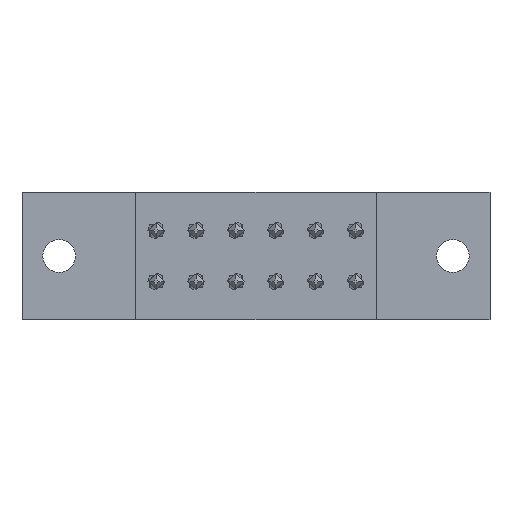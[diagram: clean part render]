
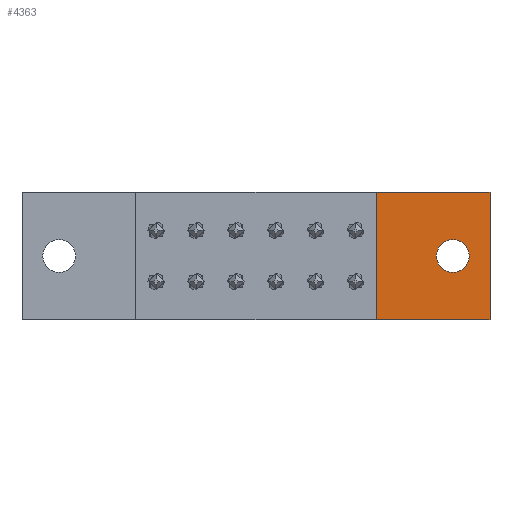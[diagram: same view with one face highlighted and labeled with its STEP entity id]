
A CAD part, front view. The second image highlights one B-rep face of the part: STEP entity #4363.
In plain terms, the highlighted planar face has unit normal (0, -1, 0).
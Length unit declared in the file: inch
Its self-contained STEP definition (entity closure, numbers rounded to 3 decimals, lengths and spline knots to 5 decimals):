
#389 = VERTEX_POINT ( 'NONE', #486 ) ;
#486 = CARTESIAN_POINT ( 'NONE',  ( 1.385, 0.163, 0. ) ) ;
#1177 = VECTOR ( 'NONE', #9337, 39.37008 ) ;
#1656 = ORIENTED_EDGE ( 'NONE', *, *, #9007, .T. ) ;
#1681 = LINE ( 'NONE', #3492, #4332 ) ;
#1894 = DIRECTION ( 'NONE',  ( 0., 0., -1. ) ) ;
#2116 = VERTEX_POINT ( 'NONE', #6419 ) ;
#2620 = VECTOR ( 'NONE', #1894, 39.37008 ) ;
#2778 = AXIS2_PLACEMENT_3D ( 'NONE', #4044, #10403, #4236 ) ;
#3349 = LINE ( 'NONE', #5354, #1177 ) ;
#3492 = CARTESIAN_POINT ( 'NONE',  ( 1.83, 0.163, -0.5 ) ) ;
#3791 = CARTESIAN_POINT ( 'NONE',  ( 1.6845, 0.163, -0.186 ) ) ;
#4044 = CARTESIAN_POINT ( 'NONE',  ( 1.6845, 0.163, -0.25 ) ) ;
#4084 = LINE ( 'NONE', #6228, #2620 ) ;
#4207 = VERTEX_POINT ( 'NONE', #5032 ) ;
#4236 = DIRECTION ( 'NONE',  ( 0., 0., -1. ) ) ;
#4332 = VECTOR ( 'NONE', #6622, 39.37008 ) ;
#4359 = CARTESIAN_POINT ( 'NONE',  ( 1.83, 0.163, 0. ) ) ;
#4363 = ADVANCED_FACE ( 'NONE', ( #11384, #7287 ), #12642, .T. ) ;
#5032 = CARTESIAN_POINT ( 'NONE',  ( 1.6845, 0.163, -0.314 ) ) ;
#5340 = DIRECTION ( 'NONE',  ( 1., 0., 0. ) ) ;
#5354 = CARTESIAN_POINT ( 'NONE',  ( 1.83, 0.163, 0. ) ) ;
#5498 = EDGE_CURVE ( 'NONE', #2116, #389, #3349, .T. ) ;
#6051 = EDGE_CURVE ( 'NONE', #7938, #4207, #7603, .T. ) ;
#6228 = CARTESIAN_POINT ( 'NONE',  ( 1.385, 0.163, -0.5 ) ) ;
#6338 = ORIENTED_EDGE ( 'NONE', *, *, #12114, .T. ) ;
#6344 = DIRECTION ( 'NONE',  ( 0., -1., 0. ) ) ;
#6419 = CARTESIAN_POINT ( 'NONE',  ( 1.83, 0.163, 0. ) ) ;
#6596 = CIRCLE ( 'NONE', #2778, 0.064 ) ;
#6622 = DIRECTION ( 'NONE',  ( 0., 0., 1. ) ) ;
#6713 = DIRECTION ( 'NONE',  ( 0., 1., 0. ) ) ;
#6801 = ORIENTED_EDGE ( 'NONE', *, *, #5498, .T. ) ;
#7287 = FACE_BOUND ( 'NONE', #12776, .T. ) ;
#7554 = ORIENTED_EDGE ( 'NONE', *, *, #12461, .T. ) ;
#7571 = DIRECTION ( 'NONE',  ( 0., 0., -1. ) ) ;
#7603 = CIRCLE ( 'NONE', #8431, 0.064 ) ;
#7763 = DIRECTION ( 'NONE',  ( 0., 0., -1. ) ) ;
#7938 = VERTEX_POINT ( 'NONE', #3791 ) ;
#8334 = AXIS2_PLACEMENT_3D ( 'NONE', #4359, #6344, #7571 ) ;
#8427 = CARTESIAN_POINT ( 'NONE',  ( 1.83, 0.163, -0.5 ) ) ;
#8431 = AXIS2_PLACEMENT_3D ( 'NONE', #9819, #6713, #7763 ) ;
#8997 = VECTOR ( 'NONE', #5340, 39.37008 ) ;
#9007 = EDGE_CURVE ( 'NONE', #9105, #2116, #1681, .T. ) ;
#9105 = VERTEX_POINT ( 'NONE', #8427 ) ;
#9337 = DIRECTION ( 'NONE',  ( -1., 0., 0. ) ) ;
#9371 = VERTEX_POINT ( 'NONE', #9833 ) ;
#9819 = CARTESIAN_POINT ( 'NONE',  ( 1.6845, 0.163, -0.25 ) ) ;
#9833 = CARTESIAN_POINT ( 'NONE',  ( 1.385, 0.163, -0.5 ) ) ;
#10403 = DIRECTION ( 'NONE',  ( 0., 1., 0. ) ) ;
#10421 = CARTESIAN_POINT ( 'NONE',  ( 1.83, 0.163, -0.5 ) ) ;
#11384 = FACE_OUTER_BOUND ( 'NONE', #11823, .T. ) ;
#11470 = EDGE_CURVE ( 'NONE', #4207, #7938, #6596, .T. ) ;
#11823 = EDGE_LOOP ( 'NONE', ( #1656, #6801, #6338, #7554 ) ) ;
#12007 = ORIENTED_EDGE ( 'NONE', *, *, #11470, .T. ) ;
#12114 = EDGE_CURVE ( 'NONE', #389, #9371, #4084, .T. ) ;
#12461 = EDGE_CURVE ( 'NONE', #9371, #9105, #13160, .T. ) ;
#12642 = PLANE ( 'NONE',  #8334 ) ;
#12776 = EDGE_LOOP ( 'NONE', ( #13578, #12007 ) ) ;
#13160 = LINE ( 'NONE', #10421, #8997 ) ;
#13578 = ORIENTED_EDGE ( 'NONE', *, *, #6051, .T. ) ;
